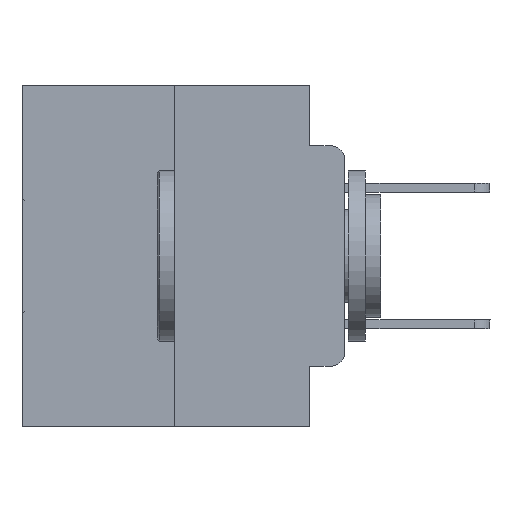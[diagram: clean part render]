
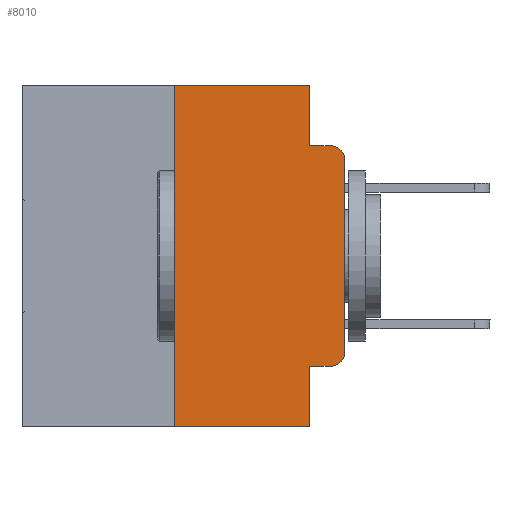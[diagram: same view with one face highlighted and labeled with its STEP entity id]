
A CAD part, left-side view. The second image highlights one B-rep face of the part: STEP entity #8010.
In plain terms, the highlighted planar face has unit normal (-1, 0, 0).
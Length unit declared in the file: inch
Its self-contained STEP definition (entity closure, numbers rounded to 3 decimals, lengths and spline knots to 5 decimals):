
#253 = FACE_OUTER_BOUND ( 'NONE', #18984, .T. ) ;
#329 = ORIENTED_EDGE ( 'NONE', *, *, #18699, .T. ) ;
#364 = LINE ( 'NONE', #9909, #13373 ) ;
#596 = DIRECTION ( 'NONE',  ( 0., -1., 0. ) ) ;
#882 = DIRECTION ( 'NONE',  ( 1., 0., 0. ) ) ;
#1208 = VECTOR ( 'NONE', #3109, 39.37008 ) ;
#1435 = ORIENTED_EDGE ( 'NONE', *, *, #23489, .T. ) ;
#1651 = ORIENTED_EDGE ( 'NONE', *, *, #26248, .F. ) ;
#1849 = CARTESIAN_POINT ( 'NONE',  ( 0., 0.051, -0.0885 ) ) ;
#1985 = CARTESIAN_POINT ( 'NONE',  ( 0., 0.02, -0.1085 ) ) ;
#2397 = AXIS2_PLACEMENT_3D ( 'NONE', #25920, #7238, #23392 ) ;
#2402 = CARTESIAN_POINT ( 'NONE',  ( 0., 0.051, -0.5 ) ) ;
#2409 = VECTOR ( 'NONE', #7210, 39.37008 ) ;
#3109 = DIRECTION ( 'NONE',  ( 0., 0., 1. ) ) ;
#3820 = VERTEX_POINT ( 'NONE', #12954 ) ;
#4769 = CARTESIAN_POINT ( 'NONE',  ( 0., 0.473, 0. ) ) ;
#5367 = VERTEX_POINT ( 'NONE', #12438 ) ;
#5700 = CIRCLE ( 'NONE', #2397, 0.02 ) ;
#6175 = VERTEX_POINT ( 'NONE', #9522 ) ;
#6411 = VECTOR ( 'NONE', #8514, 39.37008 ) ;
#6636 = AXIS2_PLACEMENT_3D ( 'NONE', #4769, #882, #28613 ) ;
#7210 = DIRECTION ( 'NONE',  ( 0., -1., 0. ) ) ;
#7238 = DIRECTION ( 'NONE',  ( -1., 0., 0. ) ) ;
#7394 = LINE ( 'NONE', #28797, #1208 ) ;
#7738 = VERTEX_POINT ( 'NONE', #25163 ) ;
#7858 = EDGE_CURVE ( 'NONE', #5367, #6175, #12570, .T. ) ;
#8010 = ADVANCED_FACE ( 'NONE', ( #253 ), #23044, .F. ) ;
#8235 = VECTOR ( 'NONE', #596, 39.37008 ) ;
#8514 = DIRECTION ( 'NONE',  ( 0., -1., 0. ) ) ;
#8924 = LINE ( 'NONE', #15657, #6411 ) ;
#9522 = CARTESIAN_POINT ( 'NONE',  ( 0., 0.25, 0. ) ) ;
#9909 = CARTESIAN_POINT ( 'NONE',  ( 0., 0.051, 0. ) ) ;
#11338 = ORIENTED_EDGE ( 'NONE', *, *, #26597, .T. ) ;
#11707 = VERTEX_POINT ( 'NONE', #24522 ) ;
#11967 = VERTEX_POINT ( 'NONE', #2402 ) ;
#11968 = DIRECTION ( 'NONE',  ( 0., 0., -1. ) ) ;
#12046 = CIRCLE ( 'NONE', #28879, 0.02 ) ;
#12438 = CARTESIAN_POINT ( 'NONE',  ( 0., 0.25, -0.5 ) ) ;
#12458 = VERTEX_POINT ( 'NONE', #1849 ) ;
#12570 = LINE ( 'NONE', #22541, #12925 ) ;
#12925 = VECTOR ( 'NONE', #22737, 39.37008 ) ;
#12954 = CARTESIAN_POINT ( 'NONE',  ( 0., 0.051, -0.4115 ) ) ;
#13373 = VECTOR ( 'NONE', #14415, 39.37008 ) ;
#13817 = CARTESIAN_POINT ( 'NONE',  ( 0., 0.051, -0.4115 ) ) ;
#14251 = VECTOR ( 'NONE', #27087, 39.37008 ) ;
#14335 = LINE ( 'NONE', #28535, #8235 ) ;
#14415 = DIRECTION ( 'NONE',  ( 0., 0., -1. ) ) ;
#14671 = CARTESIAN_POINT ( 'NONE',  ( 0., 0.02, -0.4115 ) ) ;
#15657 = CARTESIAN_POINT ( 'NONE',  ( 0., 0.473, 0. ) ) ;
#15972 = ORIENTED_EDGE ( 'NONE', *, *, #18960, .F. ) ;
#16003 = ORIENTED_EDGE ( 'NONE', *, *, #24710, .T. ) ;
#17528 = LINE ( 'NONE', #17787, #14251 ) ;
#17787 = CARTESIAN_POINT ( 'NONE',  ( 0., 0.051, -0.0885 ) ) ;
#18699 = EDGE_CURVE ( 'NONE', #24018, #11707, #12046, .T. ) ;
#18960 = EDGE_CURVE ( 'NONE', #7738, #12458, #29059, .T. ) ;
#18984 = EDGE_LOOP ( 'NONE', ( #11338, #329, #1651, #15972, #27698, #23035, #16003, #21436, #1435, #22856 ) ) ;
#19678 = EDGE_CURVE ( 'NONE', #3820, #11967, #364, .T. ) ;
#20279 = DIRECTION ( 'NONE',  ( -1., 0., 0. ) ) ;
#21185 = CARTESIAN_POINT ( 'NONE',  ( 0., 0.051, 0. ) ) ;
#21436 = ORIENTED_EDGE ( 'NONE', *, *, #19678, .F. ) ;
#22140 = VECTOR ( 'NONE', #11968, 39.37008 ) ;
#22541 = CARTESIAN_POINT ( 'NONE',  ( 0., 0.25, 0. ) ) ;
#22737 = DIRECTION ( 'NONE',  ( 0., 0., 1. ) ) ;
#22856 = ORIENTED_EDGE ( 'NONE', *, *, #23016, .T. ) ;
#23016 = EDGE_CURVE ( 'NONE', #27791, #26992, #5700, .T. ) ;
#23035 = ORIENTED_EDGE ( 'NONE', *, *, #7858, .F. ) ;
#23044 = PLANE ( 'NONE',  #6636 ) ;
#23392 = DIRECTION ( 'NONE',  ( 0., 0., -1. ) ) ;
#23489 = EDGE_CURVE ( 'NONE', #3820, #27791, #24806, .T. ) ;
#24018 = VERTEX_POINT ( 'NONE', #28671 ) ;
#24522 = CARTESIAN_POINT ( 'NONE',  ( 0., 0.02, -0.0885 ) ) ;
#24710 = EDGE_CURVE ( 'NONE', #5367, #11967, #14335, .T. ) ;
#24806 = LINE ( 'NONE', #13817, #2409 ) ;
#25103 = EDGE_CURVE ( 'NONE', #6175, #7738, #8924, .T. ) ;
#25163 = CARTESIAN_POINT ( 'NONE',  ( 0., 0.051, 0. ) ) ;
#25920 = CARTESIAN_POINT ( 'NONE',  ( 0., 0.02, -0.3915 ) ) ;
#26248 = EDGE_CURVE ( 'NONE', #12458, #11707, #17528, .T. ) ;
#26597 = EDGE_CURVE ( 'NONE', #26992, #24018, #7394, .T. ) ;
#26992 = VERTEX_POINT ( 'NONE', #27549 ) ;
#27087 = DIRECTION ( 'NONE',  ( 0., -1., 0. ) ) ;
#27549 = CARTESIAN_POINT ( 'NONE',  ( 0., 0., -0.3915 ) ) ;
#27698 = ORIENTED_EDGE ( 'NONE', *, *, #25103, .F. ) ;
#27791 = VERTEX_POINT ( 'NONE', #14671 ) ;
#28535 = CARTESIAN_POINT ( 'NONE',  ( 0., 0.473, -0.5 ) ) ;
#28613 = DIRECTION ( 'NONE',  ( 0., 0., -1. ) ) ;
#28671 = CARTESIAN_POINT ( 'NONE',  ( 0., 0., -0.1085 ) ) ;
#28797 = CARTESIAN_POINT ( 'NONE',  ( 0., 0., 0. ) ) ;
#28879 = AXIS2_PLACEMENT_3D ( 'NONE', #1985, #20279, #29755 ) ;
#29059 = LINE ( 'NONE', #21185, #22140 ) ;
#29755 = DIRECTION ( 'NONE',  ( 0., 0., -1. ) ) ;
